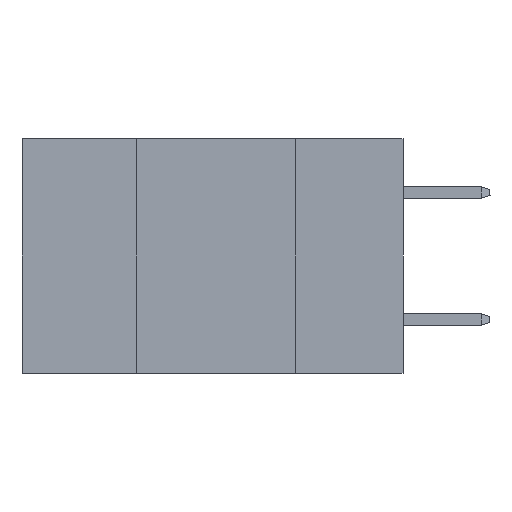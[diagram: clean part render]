
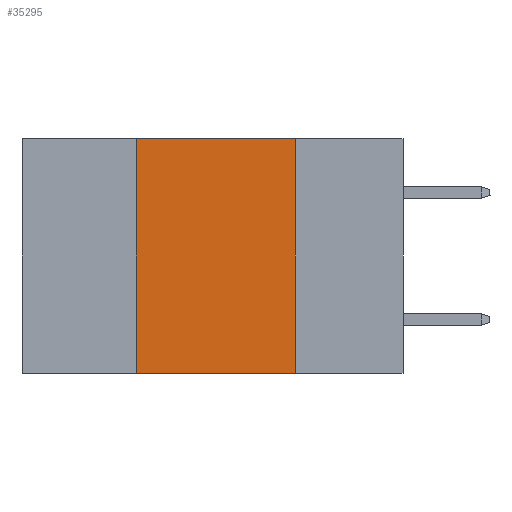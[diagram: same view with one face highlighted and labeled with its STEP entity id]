
A CAD part, left-side view. The second image highlights one B-rep face of the part: STEP entity #35295.
In plain terms, the highlighted planar face has unit normal (-1, 0, 0).
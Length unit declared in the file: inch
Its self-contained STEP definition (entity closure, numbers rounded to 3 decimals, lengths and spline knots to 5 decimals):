
#1002 = ORIENTED_EDGE ( 'NONE', *, *, #19784, .F. ) ;
#2770 = AXIS2_PLACEMENT_3D ( 'NONE', #43414, #28952, #35939 ) ;
#4076 = LINE ( 'NONE', #36549, #34451 ) ;
#6421 = VERTEX_POINT ( 'NONE', #19512 ) ;
#7030 = CARTESIAN_POINT ( 'NONE',  ( 0., 0.42, 0. ) ) ;
#7475 = ORIENTED_EDGE ( 'NONE', *, *, #25004, .F. ) ;
#8155 = EDGE_LOOP ( 'NONE', ( #1002, #37483, #7475, #19427 ) ) ;
#12032 = DIRECTION ( 'NONE',  ( 0., 0., -1. ) ) ;
#15319 = DIRECTION ( 'NONE',  ( 0., 0., 1. ) ) ;
#16585 = VERTEX_POINT ( 'NONE', #41530 ) ;
#18306 = DIRECTION ( 'NONE',  ( 0., -1., 0. ) ) ;
#18953 = CARTESIAN_POINT ( 'NONE',  ( 0., 0.17, 0. ) ) ;
#19427 = ORIENTED_EDGE ( 'NONE', *, *, #30244, .T. ) ;
#19512 = CARTESIAN_POINT ( 'NONE',  ( 0., 0.42, -0.37 ) ) ;
#19784 = EDGE_CURVE ( 'NONE', #33220, #16585, #4076, .T. ) ;
#20218 = LINE ( 'NONE', #30974, #39124 ) ;
#21701 = FACE_OUTER_BOUND ( 'NONE', #8155, .T. ) ;
#23001 = LINE ( 'NONE', #40069, #33235 ) ;
#25004 = EDGE_CURVE ( 'NONE', #6421, #25823, #23001, .T. ) ;
#25304 = EDGE_CURVE ( 'NONE', #25823, #33220, #32089, .T. ) ;
#25823 = VERTEX_POINT ( 'NONE', #7030 ) ;
#28952 = DIRECTION ( 'NONE',  ( 1., 0., 0. ) ) ;
#29053 = CARTESIAN_POINT ( 'NONE',  ( 0., 0.6, 0. ) ) ;
#30244 = EDGE_CURVE ( 'NONE', #6421, #16585, #20218, .T. ) ;
#30974 = CARTESIAN_POINT ( 'NONE',  ( 0., 0.6, -0.37 ) ) ;
#32089 = LINE ( 'NONE', #29053, #37007 ) ;
#33220 = VERTEX_POINT ( 'NONE', #18953 ) ;
#33235 = VECTOR ( 'NONE', #15319, 39.37008 ) ;
#34451 = VECTOR ( 'NONE', #12032, 39.37008 ) ;
#35295 = ADVANCED_FACE ( 'NONE', ( #21701 ), #43643, .F. ) ;
#35939 = DIRECTION ( 'NONE',  ( 0., 0., -1. ) ) ;
#36549 = CARTESIAN_POINT ( 'NONE',  ( 0., 0.17, 0. ) ) ;
#37007 = VECTOR ( 'NONE', #18306, 39.37008 ) ;
#37483 = ORIENTED_EDGE ( 'NONE', *, *, #25304, .F. ) ;
#39124 = VECTOR ( 'NONE', #41472, 39.37008 ) ;
#40069 = CARTESIAN_POINT ( 'NONE',  ( 0., 0.42, 0. ) ) ;
#41472 = DIRECTION ( 'NONE',  ( 0., -1., 0. ) ) ;
#41530 = CARTESIAN_POINT ( 'NONE',  ( 0., 0.17, -0.37 ) ) ;
#43414 = CARTESIAN_POINT ( 'NONE',  ( 0., 0.6, 0. ) ) ;
#43643 = PLANE ( 'NONE',  #2770 ) ;
